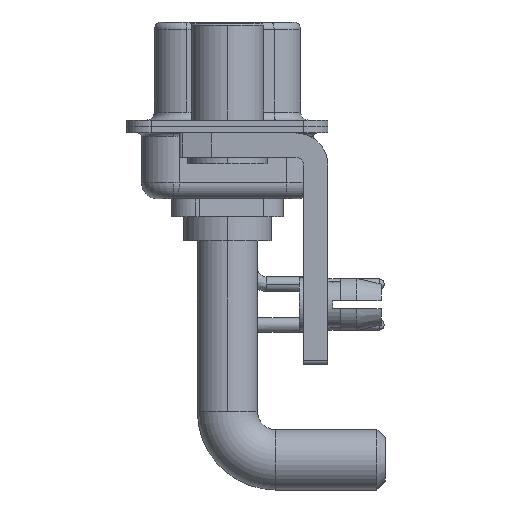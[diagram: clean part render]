
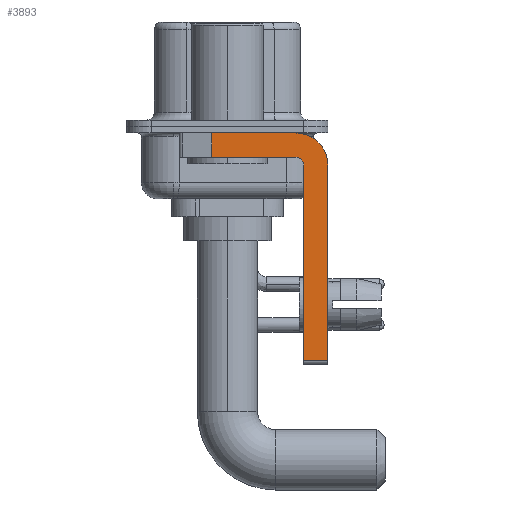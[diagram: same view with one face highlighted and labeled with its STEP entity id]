
A CAD part, left-side view. The second image highlights one B-rep face of the part: STEP entity #3893.
In plain terms, the highlighted planar face has unit normal (-1, 0, 0).
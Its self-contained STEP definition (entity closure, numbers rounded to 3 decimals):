
#79 = AXIS2_PLACEMENT_3D ( 'NONE', #26739, #5150, #15742 ) ;
#738 = EDGE_CURVE ( 'NONE', #10161, #7620, #13947, .T. ) ;
#2243 = CARTESIAN_POINT ( 'NONE',  ( -2.9, 0.978, -1.9 ) ) ;
#2664 = CARTESIAN_POINT ( 'NONE',  ( -2.9, -4.75, -14.55 ) ) ;
#2773 = DIRECTION ( 'NONE',  ( 0., 0., -1. ) ) ;
#2914 = DIRECTION ( 'NONE',  ( 1., 0., 0. ) ) ;
#3041 = AXIS2_PLACEMENT_3D ( 'NONE', #13213, #15529, #24482 ) ;
#3587 = EDGE_LOOP ( 'NONE', ( #27824, #14175, #14307, #10233, #28080, #17726, #9014, #12266 ) ) ;
#3753 = VERTEX_POINT ( 'NONE', #2243 ) ;
#3760 = LINE ( 'NONE', #21125, #26319 ) ;
#3813 = VERTEX_POINT ( 'NONE', #2664 ) ;
#3893 = ADVANCED_FACE ( 'NONE', ( #9284 ), #18112, .F. ) ;
#4054 = EDGE_CURVE ( 'NONE', #13513, #13393, #3760, .T. ) ;
#4277 = EDGE_CURVE ( 'NONE', #4643, #27381, #20380, .T. ) ;
#4643 = VERTEX_POINT ( 'NONE', #10957 ) ;
#5150 = DIRECTION ( 'NONE',  ( -1., 0., 0. ) ) ;
#5955 = EDGE_CURVE ( 'NONE', #13393, #4643, #16414, .T. ) ;
#6215 = VECTOR ( 'NONE', #16602, 1000. ) ;
#7620 = VERTEX_POINT ( 'NONE', #27799 ) ;
#8541 = CARTESIAN_POINT ( 'NONE',  ( -2.9, -6.25, -14.55 ) ) ;
#9014 = ORIENTED_EDGE ( 'NONE', *, *, #4277, .F. ) ;
#9128 = CARTESIAN_POINT ( 'NONE',  ( -2.9, -4.25, -0.4 ) ) ;
#9284 = FACE_OUTER_BOUND ( 'NONE', #3587, .T. ) ;
#10161 = VERTEX_POINT ( 'NONE', #24197 ) ;
#10233 = ORIENTED_EDGE ( 'NONE', *, *, #738, .F. ) ;
#10410 = DIRECTION ( 'NONE',  ( 0., -1., 0. ) ) ;
#10772 = EDGE_CURVE ( 'NONE', #3813, #10161, #27442, .T. ) ;
#10957 = CARTESIAN_POINT ( 'NONE',  ( -2.9, -6.25, -2.4 ) ) ;
#11858 = EDGE_CURVE ( 'NONE', #3813, #27381, #25633, .T. ) ;
#12266 = ORIENTED_EDGE ( 'NONE', *, *, #5955, .F. ) ;
#12610 = CARTESIAN_POINT ( 'NONE',  ( -2.9, -4.25, -14.55 ) ) ;
#13213 = CARTESIAN_POINT ( 'NONE',  ( -2.9, -4.25, -2.4 ) ) ;
#13393 = VERTEX_POINT ( 'NONE', #9128 ) ;
#13513 = VERTEX_POINT ( 'NONE', #20395 ) ;
#13608 = LINE ( 'NONE', #15212, #15189 ) ;
#13947 = CIRCLE ( 'NONE', #79, 0.5 ) ;
#14175 = ORIENTED_EDGE ( 'NONE', *, *, #21872, .T. ) ;
#14307 = ORIENTED_EDGE ( 'NONE', *, *, #16105, .F. ) ;
#14576 = CARTESIAN_POINT ( 'NONE',  ( -2.9, -4.75, -14.8 ) ) ;
#15189 = VECTOR ( 'NONE', #26341, 1000. ) ;
#15212 = CARTESIAN_POINT ( 'NONE',  ( -2.9, -4.25, -1.9 ) ) ;
#15529 = DIRECTION ( 'NONE',  ( 1., 0., 0. ) ) ;
#15742 = DIRECTION ( 'NONE',  ( 0., 0., 1. ) ) ;
#16105 = EDGE_CURVE ( 'NONE', #7620, #3753, #13608, .T. ) ;
#16414 = CIRCLE ( 'NONE', #3041, 2. ) ;
#16602 = DIRECTION ( 'NONE',  ( 0., 0., 1. ) ) ;
#17111 = VECTOR ( 'NONE', #18362, 1000. ) ;
#17726 = ORIENTED_EDGE ( 'NONE', *, *, #11858, .T. ) ;
#18112 = PLANE ( 'NONE',  #23071 ) ;
#18362 = DIRECTION ( 'NONE',  ( 0., 0., -1. ) ) ;
#18396 = DIRECTION ( 'NONE',  ( 0., 0., -1. ) ) ;
#19259 = DIRECTION ( 'NONE',  ( 0., -1., 0. ) ) ;
#19516 = VECTOR ( 'NONE', #2773, 1000. ) ;
#20380 = LINE ( 'NONE', #22256, #17111 ) ;
#20395 = CARTESIAN_POINT ( 'NONE',  ( -2.9, 0.978, -0.4 ) ) ;
#20552 = CARTESIAN_POINT ( 'NONE',  ( -2.9, -4.25, -2.4 ) ) ;
#20988 = VECTOR ( 'NONE', #19259, 1000. ) ;
#21125 = CARTESIAN_POINT ( 'NONE',  ( -2.9, 3., -0.4 ) ) ;
#21872 = EDGE_CURVE ( 'NONE', #13513, #3753, #27094, .T. ) ;
#22256 = CARTESIAN_POINT ( 'NONE',  ( -2.9, -6.25, -2.4 ) ) ;
#23071 = AXIS2_PLACEMENT_3D ( 'NONE', #20552, #2914, #18396 ) ;
#24197 = CARTESIAN_POINT ( 'NONE',  ( -2.9, -4.75, -2.4 ) ) ;
#24482 = DIRECTION ( 'NONE',  ( 0., 0., -1. ) ) ;
#25633 = LINE ( 'NONE', #12610, #20988 ) ;
#26319 = VECTOR ( 'NONE', #10410, 1000. ) ;
#26341 = DIRECTION ( 'NONE',  ( 0., 1., 0. ) ) ;
#26739 = CARTESIAN_POINT ( 'NONE',  ( -2.9, -4.25, -2.4 ) ) ;
#27094 = LINE ( 'NONE', #27367, #19516 ) ;
#27367 = CARTESIAN_POINT ( 'NONE',  ( -2.9, 0.978, -1.9 ) ) ;
#27381 = VERTEX_POINT ( 'NONE', #8541 ) ;
#27442 = LINE ( 'NONE', #14576, #6215 ) ;
#27799 = CARTESIAN_POINT ( 'NONE',  ( -2.9, -4.25, -1.9 ) ) ;
#27824 = ORIENTED_EDGE ( 'NONE', *, *, #4054, .F. ) ;
#28080 = ORIENTED_EDGE ( 'NONE', *, *, #10772, .F. ) ;
